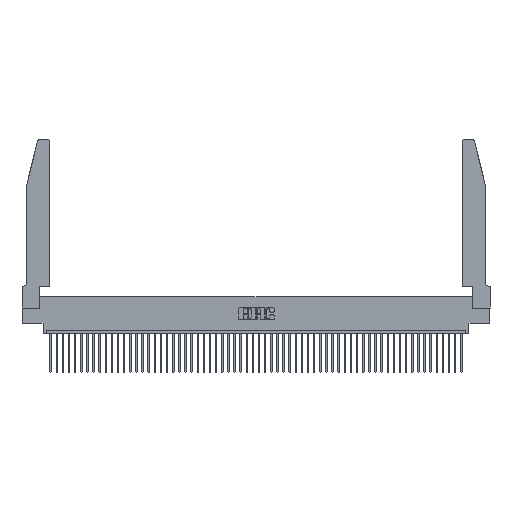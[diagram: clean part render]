
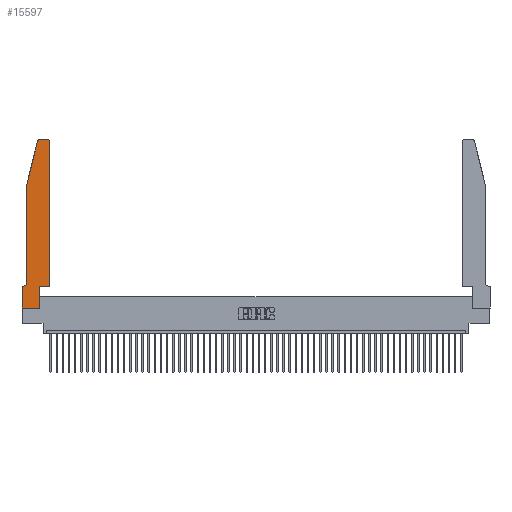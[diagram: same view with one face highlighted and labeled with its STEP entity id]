
A CAD part, top view. The second image highlights one B-rep face of the part: STEP entity #15597.
In plain terms, the highlighted planar face has unit normal (0, 0, 1).
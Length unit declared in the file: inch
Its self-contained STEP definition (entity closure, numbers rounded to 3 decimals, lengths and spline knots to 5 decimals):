
#363 = VERTEX_POINT ( 'NONE', #41210 ) ;
#368 = EDGE_CURVE ( 'NONE', #47487, #37080, #43841, .T. ) ;
#692 = DIRECTION ( 'NONE',  ( -1., 0., 0. ) ) ;
#790 = DIRECTION ( 'NONE',  ( 0., 1., 0. ) ) ;
#797 = VERTEX_POINT ( 'NONE', #47212 ) ;
#845 = CARTESIAN_POINT ( 'NONE',  ( 0.4205, 2.72, 0.37 ) ) ;
#1005 = CARTESIAN_POINT ( 'NONE',  ( 0.2605, 2.75, 0.37 ) ) ;
#1026 = DIRECTION ( 'NONE',  ( 0., 0., 1. ) ) ;
#1265 = ORIENTED_EDGE ( 'NONE', *, *, #3089, .T. ) ;
#1930 = LINE ( 'NONE', #14947, #13331 ) ;
#2095 = DIRECTION ( 'NONE',  ( 0., 1., 0. ) ) ;
#2242 = CARTESIAN_POINT ( 'NONE',  ( 0., 0., 0.37 ) ) ;
#2574 = VERTEX_POINT ( 'NONE', #11529 ) ;
#2604 = ORIENTED_EDGE ( 'NONE', *, *, #20419, .T. ) ;
#3089 = EDGE_CURVE ( 'NONE', #52318, #7483, #19516, .T. ) ;
#3547 = EDGE_CURVE ( 'NONE', #25971, #4348, #22615, .T. ) ;
#4002 = VECTOR ( 'NONE', #16551, 39.37008 ) ;
#4348 = VERTEX_POINT ( 'NONE', #28921 ) ;
#5738 = CARTESIAN_POINT ( 'NONE',  ( 0., 0.35, 0.37 ) ) ;
#7483 = VERTEX_POINT ( 'NONE', #43786 ) ;
#10847 = AXIS2_PLACEMENT_3D ( 'NONE', #34479, #38383, #22264 ) ;
#11358 = ORIENTED_EDGE ( 'NONE', *, *, #24992, .T. ) ;
#11529 = CARTESIAN_POINT ( 'NONE',  ( 0.0755, 2., 0.37 ) ) ;
#11907 = AXIS2_PLACEMENT_3D ( 'NONE', #30536, #34396, #50912 ) ;
#12461 = CARTESIAN_POINT ( 'NONE',  ( 0.0755, 2., 0.37 ) ) ;
#13195 = LINE ( 'NONE', #1005, #21457 ) ;
#13331 = VECTOR ( 'NONE', #15329, 39.37008 ) ;
#13864 = CARTESIAN_POINT ( 'NONE',  ( 0.25487, 2.72718, 0.37 ) ) ;
#14833 = LINE ( 'NONE', #12461, #4002 ) ;
#14947 = CARTESIAN_POINT ( 'NONE',  ( 0., 0., 0.37 ) ) ;
#15154 = EDGE_CURVE ( 'NONE', #44867, #52318, #30788, .T. ) ;
#15329 = DIRECTION ( 'NONE',  ( 0., -1., 0. ) ) ;
#15397 = VECTOR ( 'NONE', #18747, 39.37008 ) ;
#15597 = ADVANCED_FACE ( 'NONE', ( #31410 ), #41241, .T. ) ;
#16551 = DIRECTION ( 'NONE',  ( -0.239, -0.971, 0. ) ) ;
#17091 = EDGE_CURVE ( 'NONE', #2574, #363, #47716, .T. ) ;
#17862 = CARTESIAN_POINT ( 'NONE',  ( 0.4505, 0.35, 0.37 ) ) ;
#18581 = ORIENTED_EDGE ( 'NONE', *, *, #3547, .T. ) ;
#18747 = DIRECTION ( 'NONE',  ( 0., -1., 0. ) ) ;
#19389 = VECTOR ( 'NONE', #2095, 39.37008 ) ;
#19516 = LINE ( 'NONE', #17862, #29646 ) ;
#20419 = EDGE_CURVE ( 'NONE', #7483, #25971, #25338, .T. ) ;
#20817 = ORIENTED_EDGE ( 'NONE', *, *, #17091, .T. ) ;
#20957 = DIRECTION ( 'NONE',  ( 1., 0., 0. ) ) ;
#21087 = EDGE_CURVE ( 'NONE', #797, #44867, #50921, .T. ) ;
#21332 = CARTESIAN_POINT ( 'NONE',  ( 0.0755, 0.35, 0.37 ) ) ;
#21389 = DIRECTION ( 'NONE',  ( 1., 0., 0. ) ) ;
#21457 = VECTOR ( 'NONE', #33279, 39.37008 ) ;
#21474 = CIRCLE ( 'NONE', #11907, 0.03 ) ;
#22035 = EDGE_CURVE ( 'NONE', #37080, #797, #1930, .T. ) ;
#22264 = DIRECTION ( 'NONE',  ( 1., 0., 0. ) ) ;
#22615 = CIRCLE ( 'NONE', #45462, 0.03 ) ;
#24992 = EDGE_CURVE ( 'NONE', #363, #47487, #34008, .T. ) ;
#25338 = LINE ( 'NONE', #33462, #52061 ) ;
#25971 = VERTEX_POINT ( 'NONE', #28387 ) ;
#26336 = CARTESIAN_POINT ( 'NONE',  ( 0.0755, 2., 0.37 ) ) ;
#27540 = CARTESIAN_POINT ( 'NONE',  ( 0.0055, 0.42, 0.37 ) ) ;
#27634 = ORIENTED_EDGE ( 'NONE', *, *, #37555, .T. ) ;
#28387 = CARTESIAN_POINT ( 'NONE',  ( 0.4505, 2.72, 0.37 ) ) ;
#28921 = CARTESIAN_POINT ( 'NONE',  ( 0.4205, 2.75, 0.37 ) ) ;
#29017 = CARTESIAN_POINT ( 'NONE',  ( 0.2865, 0.35, 0.37 ) ) ;
#29251 = AXIS2_PLACEMENT_3D ( 'NONE', #27540, #48260, #43898 ) ;
#29517 = ORIENTED_EDGE ( 'NONE', *, *, #45318, .T. ) ;
#29646 = VECTOR ( 'NONE', #21389, 39.37008 ) ;
#30536 = CARTESIAN_POINT ( 'NONE',  ( 0.284, 2.72, 0.37 ) ) ;
#30788 = LINE ( 'NONE', #29017, #19389 ) ;
#31410 = FACE_OUTER_BOUND ( 'NONE', #32412, .T. ) ;
#32412 = EDGE_LOOP ( 'NONE', ( #39496, #29517, #27634, #20817, #11358, #40438, #49356, #37125, #48844, #1265, #2604, #18581 ) ) ;
#32442 = EDGE_CURVE ( 'NONE', #4348, #32691, #13195, .T. ) ;
#32691 = VERTEX_POINT ( 'NONE', #50142 ) ;
#32965 = VECTOR ( 'NONE', #692, 39.37008 ) ;
#33279 = DIRECTION ( 'NONE',  ( -1., 0., 0. ) ) ;
#33462 = CARTESIAN_POINT ( 'NONE',  ( 0.4505, 0.35, 0.37 ) ) ;
#34008 = CIRCLE ( 'NONE', #29251, 0.07 ) ;
#34396 = DIRECTION ( 'NONE',  ( 0., 0., 1. ) ) ;
#34479 = CARTESIAN_POINT ( 'NONE',  ( 0., 0.35, 0.37 ) ) ;
#35727 = VECTOR ( 'NONE', #51401, 39.37008 ) ;
#37080 = VERTEX_POINT ( 'NONE', #5738 ) ;
#37125 = ORIENTED_EDGE ( 'NONE', *, *, #21087, .T. ) ;
#37293 = CARTESIAN_POINT ( 'NONE',  ( 0.2865, 0., 0.37 ) ) ;
#37555 = EDGE_CURVE ( 'NONE', #39443, #2574, #14833, .T. ) ;
#38383 = DIRECTION ( 'NONE',  ( 0., 0., 1. ) ) ;
#39443 = VERTEX_POINT ( 'NONE', #13864 ) ;
#39496 = ORIENTED_EDGE ( 'NONE', *, *, #32442, .T. ) ;
#40438 = ORIENTED_EDGE ( 'NONE', *, *, #368, .T. ) ;
#41210 = CARTESIAN_POINT ( 'NONE',  ( 0.0755, 0.42, 0.37 ) ) ;
#41241 = PLANE ( 'NONE',  #10847 ) ;
#43786 = CARTESIAN_POINT ( 'NONE',  ( 0.4505, 0.35, 0.37 ) ) ;
#43841 = LINE ( 'NONE', #21332, #32965 ) ;
#43898 = DIRECTION ( 'NONE',  ( -1., 0., 0. ) ) ;
#44867 = VERTEX_POINT ( 'NONE', #37293 ) ;
#45093 = CARTESIAN_POINT ( 'NONE',  ( 0.2865, 0.35, 0.37 ) ) ;
#45318 = EDGE_CURVE ( 'NONE', #32691, #39443, #21474, .T. ) ;
#45462 = AXIS2_PLACEMENT_3D ( 'NONE', #845, #1026, #20957 ) ;
#47212 = CARTESIAN_POINT ( 'NONE',  ( 0., 0., 0.37 ) ) ;
#47476 = CARTESIAN_POINT ( 'NONE',  ( 0.0055, 0.35, 0.37 ) ) ;
#47487 = VERTEX_POINT ( 'NONE', #47476 ) ;
#47716 = LINE ( 'NONE', #26336, #15397 ) ;
#48260 = DIRECTION ( 'NONE',  ( 0., 0., -1. ) ) ;
#48844 = ORIENTED_EDGE ( 'NONE', *, *, #15154, .T. ) ;
#49356 = ORIENTED_EDGE ( 'NONE', *, *, #22035, .T. ) ;
#50142 = CARTESIAN_POINT ( 'NONE',  ( 0.284, 2.75, 0.37 ) ) ;
#50912 = DIRECTION ( 'NONE',  ( 1., 0., 0. ) ) ;
#50921 = LINE ( 'NONE', #2242, #35727 ) ;
#51401 = DIRECTION ( 'NONE',  ( 1., 0., 0. ) ) ;
#52061 = VECTOR ( 'NONE', #790, 39.37008 ) ;
#52318 = VERTEX_POINT ( 'NONE', #45093 ) ;
